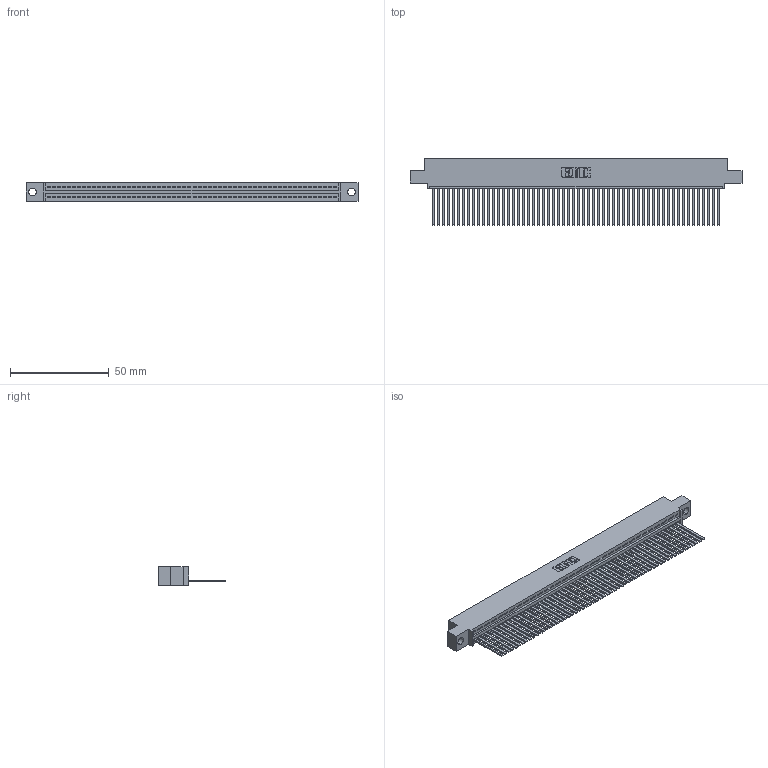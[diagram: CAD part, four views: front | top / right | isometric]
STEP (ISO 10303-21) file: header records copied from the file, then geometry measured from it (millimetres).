
FILE_DESCRIPTION (( 'STEP AP203' ), '1' );
FILE_NAME ('395-058-544-404.STEP', '2021-05-31T21:44:08', ( '' ), ( '' ), 'SwSTEP 2.0', 'SolidWorks 2020', '' );
FILE_SCHEMA (( 'CONFIG_CONTROL_DESIGN' ));
Length unit declared in the file: inch
Products named in the file (3): 345 Part_0.110 Offset - 0.156 Dia-TI; 395-058-544-404; 345-292-001_345-293-144
Assembly tree (59 placements, depth 2):
  395-058-544-404
    345 Part_0.110 Offset - 0.156 Dia-TI
    345-292-001_345-293-144  x58
Bounding box: 168.53 x 33.96 x 9.4 mm (x, y, z)
Volume: 16630.5 mm3; surface area: 24258.8 mm2
Topology: 59 solids, 59 shells, 3160 faces, 9553 edges, 6290 vertices
Faces by surface type: plane 2186, cylinder 974
Entity records: 41865 total; most frequent: CARTESIAN_POINT 7260, ORIENTED_EDGE 7250, DIRECTION 6313, EDGE_CURVE 3625, LINE 3265, VECTOR 3265, VERTEX_POINT 2414, AXIS2_PLACEMENT_3D 1524
